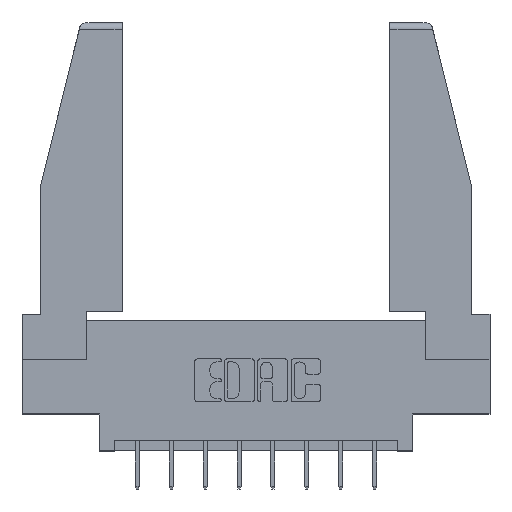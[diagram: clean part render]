
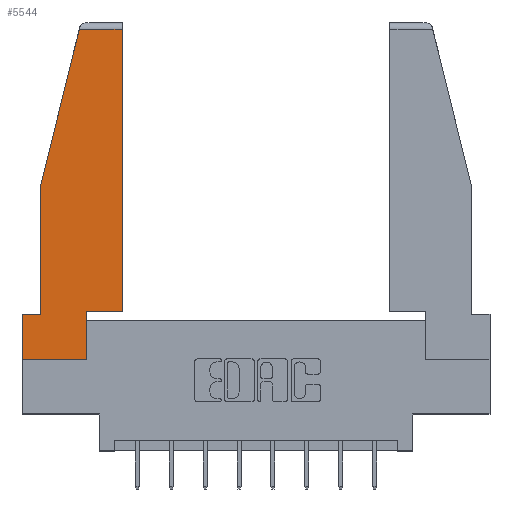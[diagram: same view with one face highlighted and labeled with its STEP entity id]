
A CAD part, top view. The second image highlights one B-rep face of the part: STEP entity #5544.
In plain terms, the highlighted planar face has unit normal (0, 0, 1).
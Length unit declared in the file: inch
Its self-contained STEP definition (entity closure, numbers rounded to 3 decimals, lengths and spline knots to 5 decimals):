
#597 = CARTESIAN_POINT ( 'NONE',  ( 0.2636, 1.52, 0. ) ) ;
#1177 = CARTESIAN_POINT ( 'NONE',  ( 0.086, 0.8, 0. ) ) ;
#1258 = EDGE_CURVE ( 'NONE', #11684, #5645, #5279, .T. ) ;
#1300 = VERTEX_POINT ( 'NONE', #597 ) ;
#1309 = EDGE_CURVE ( 'NONE', #8195, #7034, #1880, .T. ) ;
#1394 = VERTEX_POINT ( 'NONE', #4947 ) ;
#1480 = FACE_OUTER_BOUND ( 'NONE', #13111, .T. ) ;
#1582 = LINE ( 'NONE', #9699, #12831 ) ;
#1595 = DIRECTION ( 'NONE',  ( 0., -1., 0. ) ) ;
#1631 = CARTESIAN_POINT ( 'NONE',  ( 0.086, 0.8, 0. ) ) ;
#1673 = EDGE_CURVE ( 'NONE', #1394, #7425, #5297, .T. ) ;
#1812 = EDGE_CURVE ( 'NONE', #7425, #7491, #1582, .T. ) ;
#1830 = CARTESIAN_POINT ( 'NONE',  ( 0.086, 0.21, 0. ) ) ;
#1880 = LINE ( 'NONE', #1631, #7649 ) ;
#1908 = PLANE ( 'NONE',  #7512 ) ;
#3034 = CARTESIAN_POINT ( 'NONE',  ( 0.461, 1.52, 0. ) ) ;
#3198 = DIRECTION ( 'NONE',  ( 0., 1., 0. ) ) ;
#3199 = VECTOR ( 'NONE', #3198, 39.37008 ) ;
#3557 = EDGE_CURVE ( 'NONE', #7034, #11684, #5238, .T. ) ;
#3804 = DIRECTION ( 'NONE',  ( 0., 1., 0. ) ) ;
#3851 = DIRECTION ( 'NONE',  ( -1., 0., 0. ) ) ;
#3884 = VERTEX_POINT ( 'NONE', #3034 ) ;
#4013 = CARTESIAN_POINT ( 'NONE',  ( 0.297, 0.223, 0. ) ) ;
#4117 = ORIENTED_EDGE ( 'NONE', *, *, #7945, .T. ) ;
#4366 = LINE ( 'NONE', #9826, #8703 ) ;
#4398 = CARTESIAN_POINT ( 'NONE',  ( 0.297, 0., 0. ) ) ;
#4479 = ORIENTED_EDGE ( 'NONE', *, *, #3557, .T. ) ;
#4631 = DIRECTION ( 'NONE',  ( 0., -1., 0. ) ) ;
#4733 = VECTOR ( 'NONE', #9732, 39.37008 ) ;
#4794 = VECTOR ( 'NONE', #11884, 39.37008 ) ;
#4947 = CARTESIAN_POINT ( 'NONE',  ( 0.297, 0., 0. ) ) ;
#5002 = VECTOR ( 'NONE', #3851, 39.37008 ) ;
#5238 = LINE ( 'NONE', #11892, #4733 ) ;
#5279 = LINE ( 'NONE', #5711, #8946 ) ;
#5297 = LINE ( 'NONE', #4398, #3199 ) ;
#5387 = EDGE_CURVE ( 'NONE', #1300, #8195, #4366, .T. ) ;
#5544 = ADVANCED_FACE ( 'NONE', ( #1480 ), #1908, .T. ) ;
#5645 = VERTEX_POINT ( 'NONE', #11323 ) ;
#5711 = CARTESIAN_POINT ( 'NONE',  ( 0., 0.21, 0. ) ) ;
#5745 = CARTESIAN_POINT ( 'NONE',  ( 0., 1.52, 0. ) ) ;
#5913 = CARTESIAN_POINT ( 'NONE',  ( 0., 0., 0. ) ) ;
#6349 = ORIENTED_EDGE ( 'NONE', *, *, #5387, .T. ) ;
#6503 = DIRECTION ( 'NONE',  ( 1., 0., 0. ) ) ;
#6519 = CARTESIAN_POINT ( 'NONE',  ( 0., 0.21, 0. ) ) ;
#6614 = CARTESIAN_POINT ( 'NONE',  ( 0., 0., 0. ) ) ;
#6735 = LINE ( 'NONE', #6614, #4794 ) ;
#6759 = DIRECTION ( 'NONE',  ( -0.239, -0.971, 0. ) ) ;
#7015 = DIRECTION ( 'NONE',  ( 1., 0., 0. ) ) ;
#7034 = VERTEX_POINT ( 'NONE', #1830 ) ;
#7230 = ORIENTED_EDGE ( 'NONE', *, *, #1309, .T. ) ;
#7253 = EDGE_CURVE ( 'NONE', #5645, #1394, #6735, .T. ) ;
#7425 = VERTEX_POINT ( 'NONE', #4013 ) ;
#7491 = VERTEX_POINT ( 'NONE', #9402 ) ;
#7512 = AXIS2_PLACEMENT_3D ( 'NONE', #5913, #13274, #7015 ) ;
#7524 = ORIENTED_EDGE ( 'NONE', *, *, #7253, .T. ) ;
#7649 = VECTOR ( 'NONE', #4631, 39.37008 ) ;
#7742 = VECTOR ( 'NONE', #3804, 39.37008 ) ;
#7913 = ORIENTED_EDGE ( 'NONE', *, *, #1258, .T. ) ;
#7945 = EDGE_CURVE ( 'NONE', #3884, #1300, #13030, .T. ) ;
#8195 = VERTEX_POINT ( 'NONE', #1177 ) ;
#8703 = VECTOR ( 'NONE', #6759, 39.37008 ) ;
#8946 = VECTOR ( 'NONE', #1595, 39.37008 ) ;
#9402 = CARTESIAN_POINT ( 'NONE',  ( 0.461, 0.223, 0. ) ) ;
#9699 = CARTESIAN_POINT ( 'NONE',  ( 0.297, 0.223, 0. ) ) ;
#9732 = DIRECTION ( 'NONE',  ( -1., 0., 0. ) ) ;
#9826 = CARTESIAN_POINT ( 'NONE',  ( 0.271, 1.55, 0. ) ) ;
#10606 = ORIENTED_EDGE ( 'NONE', *, *, #1812, .T. ) ;
#11218 = ORIENTED_EDGE ( 'NONE', *, *, #12167, .T. ) ;
#11323 = CARTESIAN_POINT ( 'NONE',  ( 0., 0., 0. ) ) ;
#11462 = ORIENTED_EDGE ( 'NONE', *, *, #1673, .T. ) ;
#11684 = VERTEX_POINT ( 'NONE', #6519 ) ;
#11884 = DIRECTION ( 'NONE',  ( 1., 0., 0. ) ) ;
#11892 = CARTESIAN_POINT ( 'NONE',  ( 0., 0.21, 0. ) ) ;
#12167 = EDGE_CURVE ( 'NONE', #7491, #3884, #13230, .T. ) ;
#12831 = VECTOR ( 'NONE', #6503, 39.37008 ) ;
#13030 = LINE ( 'NONE', #5745, #5002 ) ;
#13111 = EDGE_LOOP ( 'NONE', ( #11218, #4117, #6349, #7230, #4479, #7913, #7524, #11462, #10606 ) ) ;
#13230 = LINE ( 'NONE', #13242, #7742 ) ;
#13242 = CARTESIAN_POINT ( 'NONE',  ( 0.461, 0.223, 0. ) ) ;
#13274 = DIRECTION ( 'NONE',  ( 0., 0., 1. ) ) ;
